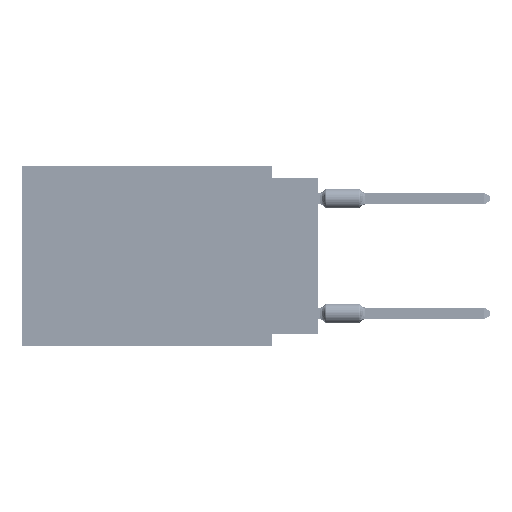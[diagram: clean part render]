
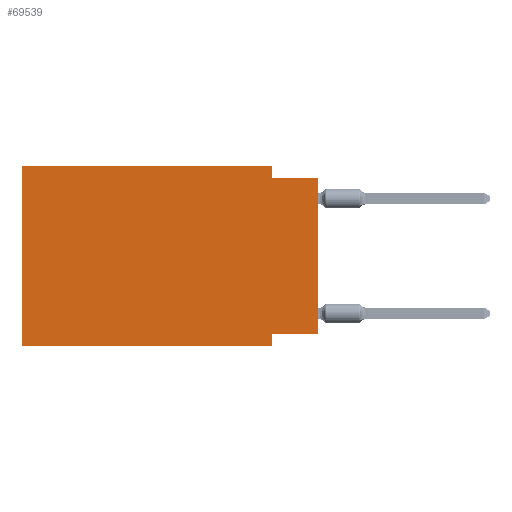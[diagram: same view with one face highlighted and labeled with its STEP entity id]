
A CAD part, left-side view. The second image highlights one B-rep face of the part: STEP entity #69539.
In plain terms, the highlighted planar face has unit normal (-1, 0, 0).
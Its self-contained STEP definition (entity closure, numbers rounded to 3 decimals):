
#658 = VERTEX_POINT ( 'NONE', #13631 ) ;
#1748 = DIRECTION ( 'NONE',  ( 1., 0., 0. ) ) ;
#2315 = LINE ( 'NONE', #59027, #81338 ) ;
#5385 = VECTOR ( 'NONE', #83002, 1000. ) ;
#10679 = EDGE_LOOP ( 'NONE', ( #68812, #63905, #29514, #42516, #57094, #52159, #59031, #42424 ) ) ;
#13171 = CARTESIAN_POINT ( 'NONE',  ( 0., 16.383, 0. ) ) ;
#13631 = CARTESIAN_POINT ( 'NONE',  ( 0., 2.54, -0.635 ) ) ;
#13681 = EDGE_CURVE ( 'NONE', #80653, #658, #2315, .T. ) ;
#16370 = VERTEX_POINT ( 'NONE', #23280 ) ;
#18325 = DIRECTION ( 'NONE',  ( 0., 0., -1. ) ) ;
#20155 = CARTESIAN_POINT ( 'NONE',  ( 0., 2.54, 0. ) ) ;
#20383 = CARTESIAN_POINT ( 'NONE',  ( 0., 2.54, -9.906 ) ) ;
#21458 = FACE_OUTER_BOUND ( 'NONE', #10679, .T. ) ;
#22164 = CARTESIAN_POINT ( 'NONE',  ( 0., 16.383, -9.906 ) ) ;
#22272 = VERTEX_POINT ( 'NONE', #20383 ) ;
#23280 = CARTESIAN_POINT ( 'NONE',  ( 0., 0., -0.635 ) ) ;
#23299 = VECTOR ( 'NONE', #55350, 1000. ) ;
#26956 = CARTESIAN_POINT ( 'NONE',  ( 0., 2.54, -9.271 ) ) ;
#29514 = ORIENTED_EDGE ( 'NONE', *, *, #13681, .F. ) ;
#32734 = EDGE_CURVE ( 'NONE', #34351, #34155, #60078, .T. ) ;
#33644 = PLANE ( 'NONE',  #54480 ) ;
#34155 = VERTEX_POINT ( 'NONE', #36101 ) ;
#34351 = VERTEX_POINT ( 'NONE', #22164 ) ;
#36101 = CARTESIAN_POINT ( 'NONE',  ( 0., 16.383, 0. ) ) ;
#36440 = CARTESIAN_POINT ( 'NONE',  ( 0., 0., -9.271 ) ) ;
#37376 = VERTEX_POINT ( 'NONE', #64991 ) ;
#38785 = DIRECTION ( 'NONE',  ( 0., -1., 0. ) ) ;
#39252 = DIRECTION ( 'NONE',  ( 0., 0., -1. ) ) ;
#40671 = EDGE_CURVE ( 'NONE', #37376, #66600, #43156, .T. ) ;
#40763 = DIRECTION ( 'NONE',  ( 0., 0., -1. ) ) ;
#42424 = ORIENTED_EDGE ( 'NONE', *, *, #40671, .F. ) ;
#42516 = ORIENTED_EDGE ( 'NONE', *, *, #69037, .F. ) ;
#43156 = LINE ( 'NONE', #36440, #23299 ) ;
#43364 = CARTESIAN_POINT ( 'NONE',  ( 0., 0., -0.635 ) ) ;
#45219 = VECTOR ( 'NONE', #38785, 1000. ) ;
#45260 = LINE ( 'NONE', #43364, #62838 ) ;
#47277 = VECTOR ( 'NONE', #56308, 1000. ) ;
#49831 = CARTESIAN_POINT ( 'NONE',  ( 0., 2.54, -9.906 ) ) ;
#50579 = LINE ( 'NONE', #13171, #45219 ) ;
#51160 = DIRECTION ( 'NONE',  ( 0., -1., 0. ) ) ;
#52159 = ORIENTED_EDGE ( 'NONE', *, *, #55975, .T. ) ;
#53760 = CARTESIAN_POINT ( 'NONE',  ( 0., 16.383, 0. ) ) ;
#54480 = AXIS2_PLACEMENT_3D ( 'NONE', #73142, #1748, #40763 ) ;
#55350 = DIRECTION ( 'NONE',  ( 0., 1., 0. ) ) ;
#55975 = EDGE_CURVE ( 'NONE', #34351, #22272, #69170, .T. ) ;
#56308 = DIRECTION ( 'NONE',  ( 0., 0., 1. ) ) ;
#56717 = CARTESIAN_POINT ( 'NONE',  ( 0., 0., 0. ) ) ;
#57094 = ORIENTED_EDGE ( 'NONE', *, *, #32734, .F. ) ;
#59027 = CARTESIAN_POINT ( 'NONE',  ( 0., 2.54, 0. ) ) ;
#59031 = ORIENTED_EDGE ( 'NONE', *, *, #82510, .F. ) ;
#60078 = LINE ( 'NONE', #53760, #68509 ) ;
#62838 = VECTOR ( 'NONE', #51160, 1000. ) ;
#62856 = CARTESIAN_POINT ( 'NONE',  ( 0., 16.383, -9.906 ) ) ;
#63731 = EDGE_CURVE ( 'NONE', #37376, #16370, #76061, .T. ) ;
#63905 = ORIENTED_EDGE ( 'NONE', *, *, #79488, .F. ) ;
#64991 = CARTESIAN_POINT ( 'NONE',  ( 0., 0., -9.271 ) ) ;
#66600 = VERTEX_POINT ( 'NONE', #26956 ) ;
#68509 = VECTOR ( 'NONE', #71452, 1000. ) ;
#68812 = ORIENTED_EDGE ( 'NONE', *, *, #63731, .T. ) ;
#69037 = EDGE_CURVE ( 'NONE', #34155, #80653, #50579, .T. ) ;
#69170 = LINE ( 'NONE', #62856, #5385 ) ;
#69539 = ADVANCED_FACE ( 'NONE', ( #21458 ), #33644, .F. ) ;
#69602 = LINE ( 'NONE', #49831, #79271 ) ;
#71452 = DIRECTION ( 'NONE',  ( 0., 0., 1. ) ) ;
#73142 = CARTESIAN_POINT ( 'NONE',  ( 0., 16.383, 0. ) ) ;
#76061 = LINE ( 'NONE', #56717, #47277 ) ;
#79271 = VECTOR ( 'NONE', #18325, 1000. ) ;
#79488 = EDGE_CURVE ( 'NONE', #658, #16370, #45260, .T. ) ;
#80653 = VERTEX_POINT ( 'NONE', #20155 ) ;
#81338 = VECTOR ( 'NONE', #39252, 1000. ) ;
#82510 = EDGE_CURVE ( 'NONE', #66600, #22272, #69602, .T. ) ;
#83002 = DIRECTION ( 'NONE',  ( 0., -1., 0. ) ) ;
